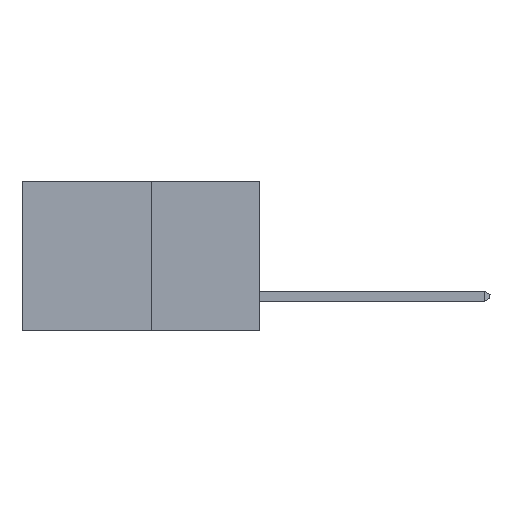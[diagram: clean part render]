
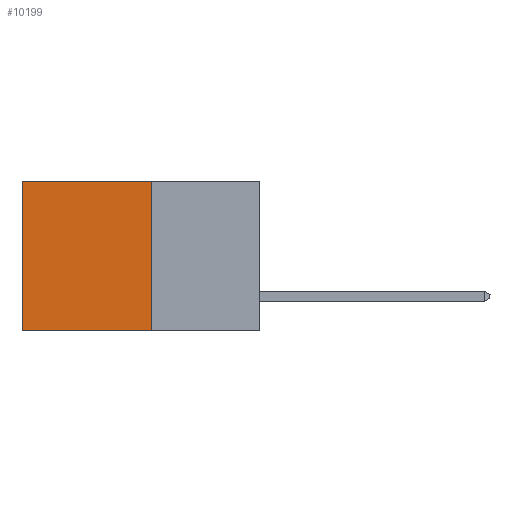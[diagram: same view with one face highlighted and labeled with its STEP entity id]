
A CAD part, left-side view. The second image highlights one B-rep face of the part: STEP entity #10199.
In plain terms, the highlighted planar face has unit normal (-1, 0, 0).
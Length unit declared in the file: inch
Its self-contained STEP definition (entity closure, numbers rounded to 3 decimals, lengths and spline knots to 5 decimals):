
#1891 = LINE ( 'NONE', #20776, #13809 ) ;
#2205 = ORIENTED_EDGE ( 'NONE', *, *, #16504, .T. ) ;
#2416 = DIRECTION ( 'NONE',  ( 0., 0., -1. ) ) ;
#3859 = CARTESIAN_POINT ( 'NONE',  ( 0.277, 0.27, 0. ) ) ;
#4995 = EDGE_CURVE ( 'NONE', #18917, #16137, #6598, .T. ) ;
#6598 = LINE ( 'NONE', #24325, #24261 ) ;
#9642 = EDGE_CURVE ( 'NONE', #16137, #11284, #1891, .T. ) ;
#10199 = ADVANCED_FACE ( 'NONE', ( #20304 ), #21429, .F. ) ;
#10530 = CARTESIAN_POINT ( 'NONE',  ( 0.277, 0.27, 0. ) ) ;
#11091 = ORIENTED_EDGE ( 'NONE', *, *, #4995, .F. ) ;
#11284 = VERTEX_POINT ( 'NONE', #22549 ) ;
#13809 = VECTOR ( 'NONE', #19931, 39.37008 ) ;
#15711 = AXIS2_PLACEMENT_3D ( 'NONE', #16738, #16098, #15777 ) ;
#15777 = DIRECTION ( 'NONE',  ( 0., 0., -1. ) ) ;
#16098 = DIRECTION ( 'NONE',  ( 1., 0., 0. ) ) ;
#16137 = VERTEX_POINT ( 'NONE', #27357 ) ;
#16479 = ORIENTED_EDGE ( 'NONE', *, *, #9642, .F. ) ;
#16504 = EDGE_CURVE ( 'NONE', #30498, #11284, #22887, .T. ) ;
#16700 = CARTESIAN_POINT ( 'NONE',  ( 0.277, 0.59, -0.37 ) ) ;
#16738 = CARTESIAN_POINT ( 'NONE',  ( 0.277, 0.27, -0.37 ) ) ;
#17231 = VECTOR ( 'NONE', #2416, 39.37008 ) ;
#18204 = VECTOR ( 'NONE', #29827, 39.37008 ) ;
#18788 = EDGE_CURVE ( 'NONE', #18917, #30498, #18968, .T. ) ;
#18917 = VERTEX_POINT ( 'NONE', #3859 ) ;
#18968 = LINE ( 'NONE', #10530, #18204 ) ;
#19448 = CARTESIAN_POINT ( 'NONE',  ( 0.277, 0.59, 0. ) ) ;
#19931 = DIRECTION ( 'NONE',  ( 0., 1., 0. ) ) ;
#20304 = FACE_OUTER_BOUND ( 'NONE', #30219, .T. ) ;
#20776 = CARTESIAN_POINT ( 'NONE',  ( 0.277, 0.27, -0.37 ) ) ;
#21429 = PLANE ( 'NONE',  #15711 ) ;
#22549 = CARTESIAN_POINT ( 'NONE',  ( 0.277, 0.59, -0.37 ) ) ;
#22887 = LINE ( 'NONE', #16700, #17231 ) ;
#24261 = VECTOR ( 'NONE', #30865, 39.37008 ) ;
#24325 = CARTESIAN_POINT ( 'NONE',  ( 0.277, 0.27, -0.37 ) ) ;
#27048 = ORIENTED_EDGE ( 'NONE', *, *, #18788, .T. ) ;
#27357 = CARTESIAN_POINT ( 'NONE',  ( 0.277, 0.27, -0.37 ) ) ;
#29827 = DIRECTION ( 'NONE',  ( 0., 1., 0. ) ) ;
#30219 = EDGE_LOOP ( 'NONE', ( #2205, #16479, #11091, #27048 ) ) ;
#30498 = VERTEX_POINT ( 'NONE', #19448 ) ;
#30865 = DIRECTION ( 'NONE',  ( 0., 0., -1. ) ) ;
